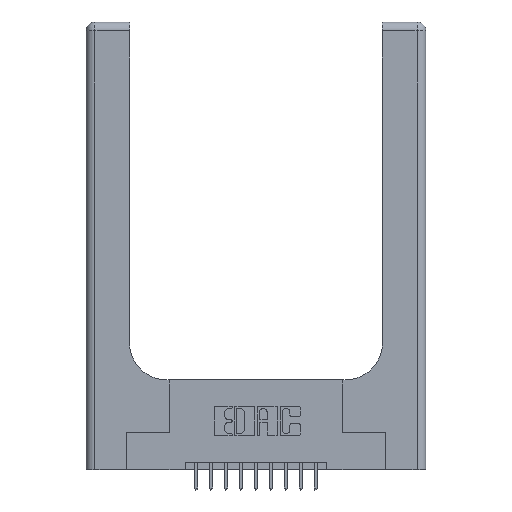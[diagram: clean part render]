
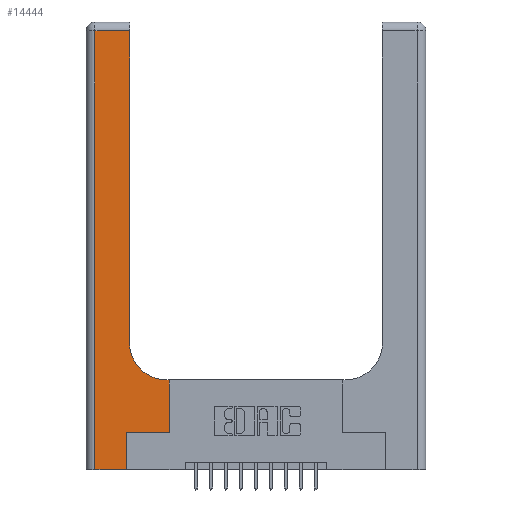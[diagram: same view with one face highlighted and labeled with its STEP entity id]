
A CAD part, top view. The second image highlights one B-rep face of the part: STEP entity #14444.
In plain terms, the highlighted planar face has unit normal (0, 0, 1).
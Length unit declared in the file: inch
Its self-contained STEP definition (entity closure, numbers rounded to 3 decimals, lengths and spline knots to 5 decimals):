
#141 = DIRECTION ( 'NONE',  ( -1., 0., 0. ) ) ;
#259 = ORIENTED_EDGE ( 'NONE', *, *, #7202, .T. ) ;
#349 = VERTEX_POINT ( 'NONE', #7556 ) ;
#437 = EDGE_CURVE ( 'NONE', #11628, #4481, #8061, .T. ) ;
#657 = ORIENTED_EDGE ( 'NONE', *, *, #437, .T. ) ;
#1105 = DIRECTION ( 'NONE',  ( 0., -1., 0. ) ) ;
#1346 = CARTESIAN_POINT ( 'NONE',  ( 0.2915, 0.85, 0.37 ) ) ;
#1969 = DIRECTION ( 'NONE',  ( 0., 1., 0. ) ) ;
#2009 = VECTOR ( 'NONE', #1969, 39.37008 ) ;
#2400 = ORIENTED_EDGE ( 'NONE', *, *, #14446, .T. ) ;
#2476 = CARTESIAN_POINT ( 'NONE',  ( 0.2915, 0.6, 0.37 ) ) ;
#2546 = FACE_OUTER_BOUND ( 'NONE', #13804, .T. ) ;
#2626 = VECTOR ( 'NONE', #13519, 39.37008 ) ;
#2798 = EDGE_CURVE ( 'NONE', #14171, #16598, #6916, .T. ) ;
#2824 = CARTESIAN_POINT ( 'NONE',  ( 0.06, 2.94, 0.37 ) ) ;
#3115 = VERTEX_POINT ( 'NONE', #9051 ) ;
#3531 = DIRECTION ( 'NONE',  ( 1., 0., 0. ) ) ;
#3674 = CARTESIAN_POINT ( 'NONE',  ( 0.269, 0., 0.37 ) ) ;
#3714 = DIRECTION ( 'NONE',  ( 0., 1., 0. ) ) ;
#3916 = VECTOR ( 'NONE', #1105, 39.37008 ) ;
#4347 = ORIENTED_EDGE ( 'NONE', *, *, #10283, .T. ) ;
#4366 = VERTEX_POINT ( 'NONE', #12750 ) ;
#4481 = VERTEX_POINT ( 'NONE', #1346 ) ;
#5447 = CARTESIAN_POINT ( 'NONE',  ( 0.5585, 0.25, 0.37 ) ) ;
#5799 = CARTESIAN_POINT ( 'NONE',  ( 0.269, 0.25, 0.37 ) ) ;
#5875 = VECTOR ( 'NONE', #3714, 39.37008 ) ;
#6116 = LINE ( 'NONE', #8707, #5875 ) ;
#6610 = ORIENTED_EDGE ( 'NONE', *, *, #14026, .T. ) ;
#6916 = LINE ( 'NONE', #5799, #2626 ) ;
#6962 = AXIS2_PLACEMENT_3D ( 'NONE', #11368, #15165, #3531 ) ;
#7202 = EDGE_CURVE ( 'NONE', #3115, #11628, #16659, .T. ) ;
#7356 = VERTEX_POINT ( 'NONE', #2824 ) ;
#7556 = CARTESIAN_POINT ( 'NONE',  ( 0.2915, 2.94, 0.37 ) ) ;
#7591 = CARTESIAN_POINT ( 'NONE',  ( 0.06, 3., 0.37 ) ) ;
#8061 = CIRCLE ( 'NONE', #6962, 0.25 ) ;
#8339 = CARTESIAN_POINT ( 'NONE',  ( 0.5415, 0.6, 0.37 ) ) ;
#8415 = VERTEX_POINT ( 'NONE', #3674 ) ;
#8471 = LINE ( 'NONE', #13606, #2009 ) ;
#8540 = ORIENTED_EDGE ( 'NONE', *, *, #16274, .T. ) ;
#8707 = CARTESIAN_POINT ( 'NONE',  ( 0.269, 0., 0.37 ) ) ;
#8724 = DIRECTION ( 'NONE',  ( -1., 0., 0. ) ) ;
#9051 = CARTESIAN_POINT ( 'NONE',  ( 0.5585, 0.6, 0.37 ) ) ;
#10190 = CARTESIAN_POINT ( 'NONE',  ( 0., 3., 0.37 ) ) ;
#10283 = EDGE_CURVE ( 'NONE', #16598, #3115, #12630, .T. ) ;
#10300 = DIRECTION ( 'NONE',  ( 1., 0., 0. ) ) ;
#10459 = AXIS2_PLACEMENT_3D ( 'NONE', #10190, #13837, #16564 ) ;
#10725 = CARTESIAN_POINT ( 'NONE',  ( 0.269, 0.25, 0.37 ) ) ;
#11368 = CARTESIAN_POINT ( 'NONE',  ( 0.5415, 0.85, 0.37 ) ) ;
#11436 = VECTOR ( 'NONE', #8724, 39.37008 ) ;
#11628 = VERTEX_POINT ( 'NONE', #8339 ) ;
#11784 = CARTESIAN_POINT ( 'NONE',  ( 0.5585, 0.25, 0.37 ) ) ;
#12306 = VECTOR ( 'NONE', #141, 39.37008 ) ;
#12630 = LINE ( 'NONE', #11784, #14167 ) ;
#12737 = LINE ( 'NONE', #7591, #3916 ) ;
#12750 = CARTESIAN_POINT ( 'NONE',  ( 0.06, 0., 0.37 ) ) ;
#12923 = LINE ( 'NONE', #14184, #13678 ) ;
#12975 = DIRECTION ( 'NONE',  ( 0., 1., 0. ) ) ;
#13519 = DIRECTION ( 'NONE',  ( 1., 0., 0. ) ) ;
#13606 = CARTESIAN_POINT ( 'NONE',  ( 0.2915, 3., 0.37 ) ) ;
#13678 = VECTOR ( 'NONE', #10300, 39.37008 ) ;
#13804 = EDGE_LOOP ( 'NONE', ( #15114, #14783, #2400, #6610, #8540, #15318, #4347, #259, #657 ) ) ;
#13831 = EDGE_CURVE ( 'NONE', #349, #7356, #14399, .T. ) ;
#13837 = DIRECTION ( 'NONE',  ( 0., 0., -1. ) ) ;
#13989 = EDGE_CURVE ( 'NONE', #4481, #349, #8471, .T. ) ;
#14026 = EDGE_CURVE ( 'NONE', #4366, #8415, #12923, .T. ) ;
#14167 = VECTOR ( 'NONE', #12975, 39.37008 ) ;
#14171 = VERTEX_POINT ( 'NONE', #10725 ) ;
#14184 = CARTESIAN_POINT ( 'NONE',  ( 0., 0., 0.37 ) ) ;
#14399 = LINE ( 'NONE', #14480, #12306 ) ;
#14444 = ADVANCED_FACE ( 'NONE', ( #2546 ), #15196, .F. ) ;
#14446 = EDGE_CURVE ( 'NONE', #7356, #4366, #12737, .T. ) ;
#14480 = CARTESIAN_POINT ( 'NONE',  ( 0., 2.94, 0.37 ) ) ;
#14783 = ORIENTED_EDGE ( 'NONE', *, *, #13831, .T. ) ;
#15114 = ORIENTED_EDGE ( 'NONE', *, *, #13989, .T. ) ;
#15165 = DIRECTION ( 'NONE',  ( 0., 0., -1. ) ) ;
#15196 = PLANE ( 'NONE',  #10459 ) ;
#15318 = ORIENTED_EDGE ( 'NONE', *, *, #2798, .T. ) ;
#16274 = EDGE_CURVE ( 'NONE', #8415, #14171, #6116, .T. ) ;
#16564 = DIRECTION ( 'NONE',  ( -1., 0., 0. ) ) ;
#16598 = VERTEX_POINT ( 'NONE', #5447 ) ;
#16659 = LINE ( 'NONE', #2476, #11436 ) ;
